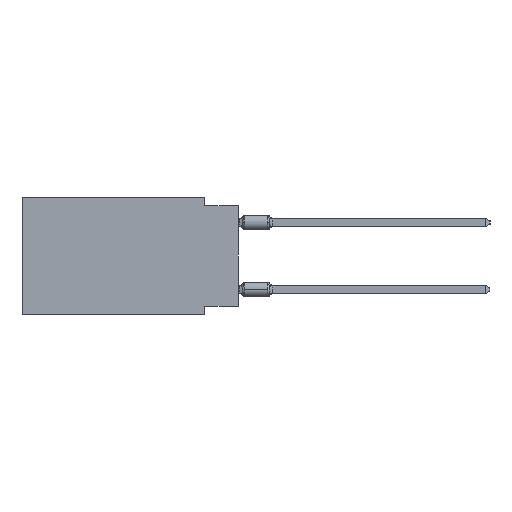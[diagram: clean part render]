
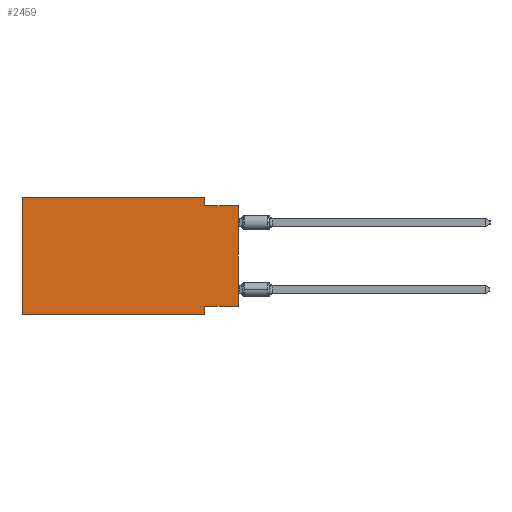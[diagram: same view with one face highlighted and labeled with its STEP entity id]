
A CAD part, left-side view. The second image highlights one B-rep face of the part: STEP entity #2459.
In plain terms, the highlighted planar face has unit normal (-1, 0, 0).
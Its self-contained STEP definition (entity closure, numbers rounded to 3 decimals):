
#209 = DIRECTION ( 'NONE',  ( 0., 0., -1. ) ) ;
#2459 = ADVANCED_FACE ( 'NONE', ( #32910 ), #40978, .F. ) ;
#2724 = AXIS2_PLACEMENT_3D ( 'NONE', #21551, #48076, #6365 ) ;
#3014 = CARTESIAN_POINT ( 'NONE',  ( 0., 16.383, -8.89 ) ) ;
#3829 = ORIENTED_EDGE ( 'NONE', *, *, #24736, .F. ) ;
#3871 = ORIENTED_EDGE ( 'NONE', *, *, #21504, .F. ) ;
#4649 = CARTESIAN_POINT ( 'NONE',  ( 0., 2.54, 0. ) ) ;
#4747 = CARTESIAN_POINT ( 'NONE',  ( 0., 2.54, -8.89 ) ) ;
#5838 = EDGE_CURVE ( 'NONE', #16451, #36805, #28060, .T. ) ;
#6365 = DIRECTION ( 'NONE',  ( 0., 0., -1. ) ) ;
#6410 = CARTESIAN_POINT ( 'NONE',  ( 0., 16.383, 0. ) ) ;
#6463 = DIRECTION ( 'NONE',  ( 0., 1., 0. ) ) ;
#7755 = CARTESIAN_POINT ( 'NONE',  ( 0., 2.54, 0. ) ) ;
#9445 = ORIENTED_EDGE ( 'NONE', *, *, #45951, .T. ) ;
#10817 = VERTEX_POINT ( 'NONE', #20480 ) ;
#12429 = VECTOR ( 'NONE', #6463, 1000. ) ;
#12552 = VERTEX_POINT ( 'NONE', #43714 ) ;
#14532 = CARTESIAN_POINT ( 'NONE',  ( 0., 0., -8.255 ) ) ;
#16096 = LINE ( 'NONE', #42629, #30239 ) ;
#16451 = VERTEX_POINT ( 'NONE', #3014 ) ;
#17402 = VERTEX_POINT ( 'NONE', #49876 ) ;
#18577 = CARTESIAN_POINT ( 'NONE',  ( 0., 0., -0.635 ) ) ;
#20480 = CARTESIAN_POINT ( 'NONE',  ( 0., 0., -8.255 ) ) ;
#21504 = EDGE_CURVE ( 'NONE', #17402, #12552, #31034, .T. ) ;
#21551 = CARTESIAN_POINT ( 'NONE',  ( 0., 16.383, 0. ) ) ;
#21890 = CARTESIAN_POINT ( 'NONE',  ( 0., 16.383, 0. ) ) ;
#23237 = CARTESIAN_POINT ( 'NONE',  ( 0., 2.54, -0.635 ) ) ;
#24272 = CARTESIAN_POINT ( 'NONE',  ( 0., 16.383, 0. ) ) ;
#24736 = EDGE_CURVE ( 'NONE', #36805, #35251, #41019, .T. ) ;
#25265 = DIRECTION ( 'NONE',  ( 0., 0., 1. ) ) ;
#25623 = VECTOR ( 'NONE', #43311, 1000. ) ;
#27909 = LINE ( 'NONE', #4649, #25623 ) ;
#27984 = DIRECTION ( 'NONE',  ( 0., -1., 0. ) ) ;
#28060 = LINE ( 'NONE', #24272, #42359 ) ;
#28090 = VECTOR ( 'NONE', #209, 1000. ) ;
#29066 = LINE ( 'NONE', #44478, #38462 ) ;
#30239 = VECTOR ( 'NONE', #27984, 1000. ) ;
#31034 = LINE ( 'NONE', #4747, #28090 ) ;
#32072 = VERTEX_POINT ( 'NONE', #18577 ) ;
#32910 = FACE_OUTER_BOUND ( 'NONE', #47184, .T. ) ;
#33016 = LINE ( 'NONE', #48189, #41744 ) ;
#33082 = EDGE_CURVE ( 'NONE', #10817, #17402, #48426, .T. ) ;
#33849 = ORIENTED_EDGE ( 'NONE', *, *, #33082, .F. ) ;
#35251 = VERTEX_POINT ( 'NONE', #7755 ) ;
#35321 = EDGE_CURVE ( 'NONE', #16451, #12552, #16096, .T. ) ;
#36805 = VERTEX_POINT ( 'NONE', #21890 ) ;
#37241 = DIRECTION ( 'NONE',  ( 0., -1., 0. ) ) ;
#38113 = EDGE_CURVE ( 'NONE', #43582, #32072, #33016, .T. ) ;
#38462 = VECTOR ( 'NONE', #25265, 1000. ) ;
#39666 = DIRECTION ( 'NONE',  ( 0., 0., 1. ) ) ;
#39938 = ORIENTED_EDGE ( 'NONE', *, *, #47128, .F. ) ;
#40978 = PLANE ( 'NONE',  #2724 ) ;
#41019 = LINE ( 'NONE', #6410, #43638 ) ;
#41744 = VECTOR ( 'NONE', #44632, 1000. ) ;
#42359 = VECTOR ( 'NONE', #39666, 1000. ) ;
#42629 = CARTESIAN_POINT ( 'NONE',  ( 0., 16.383, -8.89 ) ) ;
#42701 = ORIENTED_EDGE ( 'NONE', *, *, #38113, .F. ) ;
#43311 = DIRECTION ( 'NONE',  ( 0., 0., -1. ) ) ;
#43582 = VERTEX_POINT ( 'NONE', #23237 ) ;
#43638 = VECTOR ( 'NONE', #37241, 1000. ) ;
#43714 = CARTESIAN_POINT ( 'NONE',  ( 0., 2.54, -8.89 ) ) ;
#44478 = CARTESIAN_POINT ( 'NONE',  ( 0., 0., 0. ) ) ;
#44632 = DIRECTION ( 'NONE',  ( 0., -1., 0. ) ) ;
#45471 = ORIENTED_EDGE ( 'NONE', *, *, #35321, .T. ) ;
#45951 = EDGE_CURVE ( 'NONE', #10817, #32072, #29066, .T. ) ;
#47128 = EDGE_CURVE ( 'NONE', #35251, #43582, #27909, .T. ) ;
#47184 = EDGE_LOOP ( 'NONE', ( #9445, #42701, #39938, #3829, #48737, #45471, #3871, #33849 ) ) ;
#48076 = DIRECTION ( 'NONE',  ( 1., 0., 0. ) ) ;
#48189 = CARTESIAN_POINT ( 'NONE',  ( 0., 0., -0.635 ) ) ;
#48426 = LINE ( 'NONE', #14532, #12429 ) ;
#48737 = ORIENTED_EDGE ( 'NONE', *, *, #5838, .F. ) ;
#49876 = CARTESIAN_POINT ( 'NONE',  ( 0., 2.54, -8.255 ) ) ;
